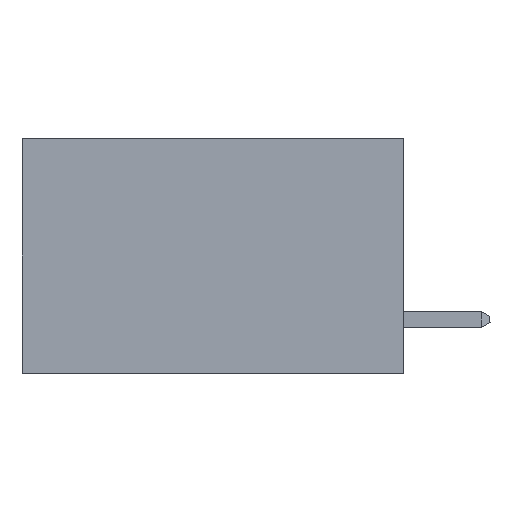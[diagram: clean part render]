
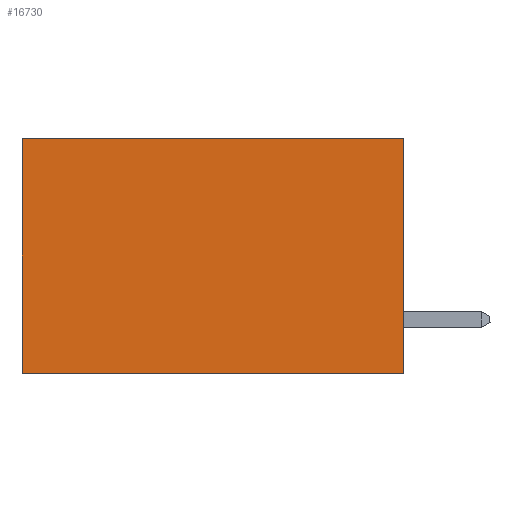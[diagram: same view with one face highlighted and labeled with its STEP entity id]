
A CAD part, left-side view. The second image highlights one B-rep face of the part: STEP entity #16730.
In plain terms, the highlighted planar face has unit normal (-1, 0, 0).
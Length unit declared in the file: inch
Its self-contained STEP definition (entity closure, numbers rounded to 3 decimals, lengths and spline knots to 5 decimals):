
#1136 = CARTESIAN_POINT ( 'NONE',  ( 0.2875, 0.6, 0. ) ) ;
#1230 = FACE_OUTER_BOUND ( 'NONE', #7943, .T. ) ;
#1925 = VERTEX_POINT ( 'NONE', #6073 ) ;
#2738 = EDGE_CURVE ( 'NONE', #1925, #16175, #5341, .T. ) ;
#2958 = DIRECTION ( 'NONE',  ( 1., 0., 0. ) ) ;
#3119 = LINE ( 'NONE', #6929, #5201 ) ;
#3268 = VERTEX_POINT ( 'NONE', #15220 ) ;
#3825 = VECTOR ( 'NONE', #6147, 39.37008 ) ;
#4246 = CARTESIAN_POINT ( 'NONE',  ( 0.2875, 0.6, -0.37 ) ) ;
#4493 = DIRECTION ( 'NONE',  ( 0., 0., -1. ) ) ;
#5201 = VECTOR ( 'NONE', #12817, 39.37008 ) ;
#5341 = LINE ( 'NONE', #10951, #15675 ) ;
#6073 = CARTESIAN_POINT ( 'NONE',  ( 0.2875, 0., 0. ) ) ;
#6147 = DIRECTION ( 'NONE',  ( 0., 0., -1. ) ) ;
#6350 = EDGE_CURVE ( 'NONE', #3268, #10966, #13458, .T. ) ;
#6437 = EDGE_CURVE ( 'NONE', #1925, #3268, #7727, .T. ) ;
#6929 = CARTESIAN_POINT ( 'NONE',  ( 0.2875, 0.6, 0. ) ) ;
#7358 = CARTESIAN_POINT ( 'NONE',  ( 0.2875, 0., 0. ) ) ;
#7546 = CARTESIAN_POINT ( 'NONE',  ( 0.2875, 0., 0. ) ) ;
#7727 = LINE ( 'NONE', #7358, #3825 ) ;
#7943 = EDGE_LOOP ( 'NONE', ( #9109, #9253, #17712, #18935 ) ) ;
#9109 = ORIENTED_EDGE ( 'NONE', *, *, #9771, .T. ) ;
#9253 = ORIENTED_EDGE ( 'NONE', *, *, #6350, .F. ) ;
#9577 = VECTOR ( 'NONE', #17309, 39.37008 ) ;
#9771 = EDGE_CURVE ( 'NONE', #16175, #10966, #3119, .T. ) ;
#10951 = CARTESIAN_POINT ( 'NONE',  ( 0.2875, 0., 0. ) ) ;
#10966 = VERTEX_POINT ( 'NONE', #4246 ) ;
#12817 = DIRECTION ( 'NONE',  ( 0., 0., -1. ) ) ;
#13283 = AXIS2_PLACEMENT_3D ( 'NONE', #7546, #2958, #4493 ) ;
#13458 = LINE ( 'NONE', #15903, #9577 ) ;
#15220 = CARTESIAN_POINT ( 'NONE',  ( 0.2875, 0., -0.37 ) ) ;
#15675 = VECTOR ( 'NONE', #16821, 39.37008 ) ;
#15903 = CARTESIAN_POINT ( 'NONE',  ( 0.2875, 0., -0.37 ) ) ;
#16123 = PLANE ( 'NONE',  #13283 ) ;
#16175 = VERTEX_POINT ( 'NONE', #1136 ) ;
#16730 = ADVANCED_FACE ( 'NONE', ( #1230 ), #16123, .F. ) ;
#16821 = DIRECTION ( 'NONE',  ( 0., 1., 0. ) ) ;
#17309 = DIRECTION ( 'NONE',  ( 0., 1., 0. ) ) ;
#17712 = ORIENTED_EDGE ( 'NONE', *, *, #6437, .F. ) ;
#18935 = ORIENTED_EDGE ( 'NONE', *, *, #2738, .T. ) ;
